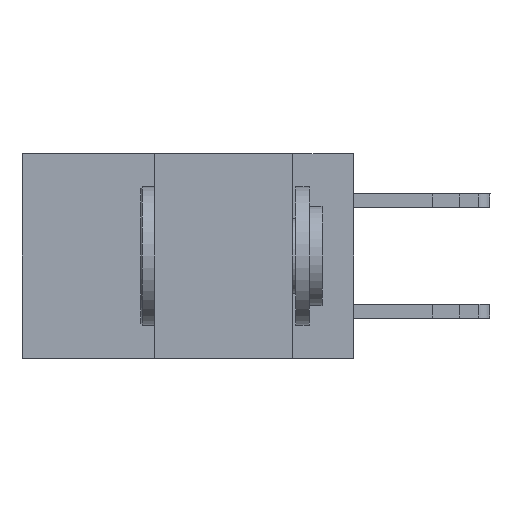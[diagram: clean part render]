
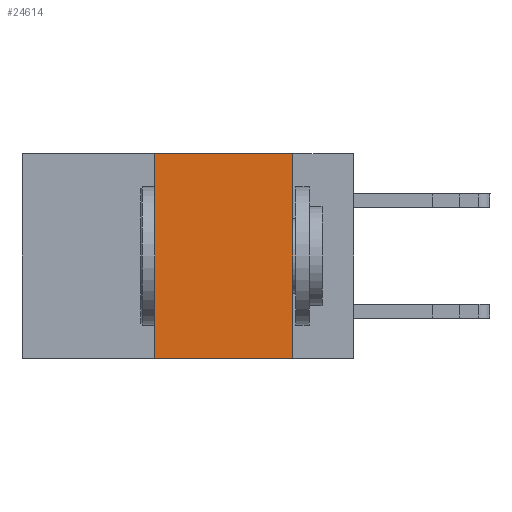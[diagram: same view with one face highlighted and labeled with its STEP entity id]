
A CAD part, left-side view. The second image highlights one B-rep face of the part: STEP entity #24614.
In plain terms, the highlighted planar face has unit normal (-1, 0, 0).
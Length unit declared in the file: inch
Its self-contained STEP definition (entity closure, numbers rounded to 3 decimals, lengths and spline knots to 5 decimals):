
#736 = DIRECTION ( 'NONE',  ( 0., -1., 0. ) ) ;
#2960 = ORIENTED_EDGE ( 'NONE', *, *, #7309, .F. ) ;
#3145 = CARTESIAN_POINT ( 'NONE',  ( 0., 0.11, 0. ) ) ;
#3205 = VECTOR ( 'NONE', #736, 39.37008 ) ;
#5243 = PLANE ( 'NONE',  #21069 ) ;
#5298 = LINE ( 'NONE', #3145, #18389 ) ;
#5333 = CARTESIAN_POINT ( 'NONE',  ( 0., 0.6, 0. ) ) ;
#5946 = VERTEX_POINT ( 'NONE', #16282 ) ;
#6484 = EDGE_CURVE ( 'NONE', #5946, #16946, #21187, .T. ) ;
#7053 = ORIENTED_EDGE ( 'NONE', *, *, #6484, .T. ) ;
#7248 = LINE ( 'NONE', #21633, #9366 ) ;
#7309 = EDGE_CURVE ( 'NONE', #25027, #16946, #5298, .T. ) ;
#8357 = CARTESIAN_POINT ( 'NONE',  ( 0., 0.11, -0.37 ) ) ;
#8451 = CARTESIAN_POINT ( 'NONE',  ( 0., 0.6, -0.37 ) ) ;
#8850 = DIRECTION ( 'NONE',  ( 1., 0., 0. ) ) ;
#9366 = VECTOR ( 'NONE', #19769, 39.37008 ) ;
#10776 = FACE_OUTER_BOUND ( 'NONE', #12259, .T. ) ;
#12187 = EDGE_CURVE ( 'NONE', #15552, #25027, #7248, .T. ) ;
#12220 = VECTOR ( 'NONE', #13065, 39.37008 ) ;
#12259 = EDGE_LOOP ( 'NONE', ( #2960, #15088, #18919, #7053 ) ) ;
#13065 = DIRECTION ( 'NONE',  ( 0., 0., 1. ) ) ;
#13392 = CARTESIAN_POINT ( 'NONE',  ( 0., 0.36, 0. ) ) ;
#15088 = ORIENTED_EDGE ( 'NONE', *, *, #12187, .F. ) ;
#15552 = VERTEX_POINT ( 'NONE', #13392 ) ;
#16282 = CARTESIAN_POINT ( 'NONE',  ( 0., 0.36, -0.37 ) ) ;
#16946 = VERTEX_POINT ( 'NONE', #8357 ) ;
#16961 = CARTESIAN_POINT ( 'NONE',  ( 0., 0.36, 0. ) ) ;
#17213 = DIRECTION ( 'NONE',  ( 0., 0., -1. ) ) ;
#18376 = EDGE_CURVE ( 'NONE', #5946, #15552, #21941, .T. ) ;
#18389 = VECTOR ( 'NONE', #17213, 39.37008 ) ;
#18919 = ORIENTED_EDGE ( 'NONE', *, *, #18376, .F. ) ;
#19769 = DIRECTION ( 'NONE',  ( 0., -1., 0. ) ) ;
#20455 = CARTESIAN_POINT ( 'NONE',  ( 0., 0.11, 0. ) ) ;
#20469 = DIRECTION ( 'NONE',  ( 0., 0., -1. ) ) ;
#21069 = AXIS2_PLACEMENT_3D ( 'NONE', #5333, #8850, #20469 ) ;
#21187 = LINE ( 'NONE', #8451, #3205 ) ;
#21633 = CARTESIAN_POINT ( 'NONE',  ( 0., 0.6, 0. ) ) ;
#21941 = LINE ( 'NONE', #16961, #12220 ) ;
#24614 = ADVANCED_FACE ( 'NONE', ( #10776 ), #5243, .F. ) ;
#25027 = VERTEX_POINT ( 'NONE', #20455 ) ;
